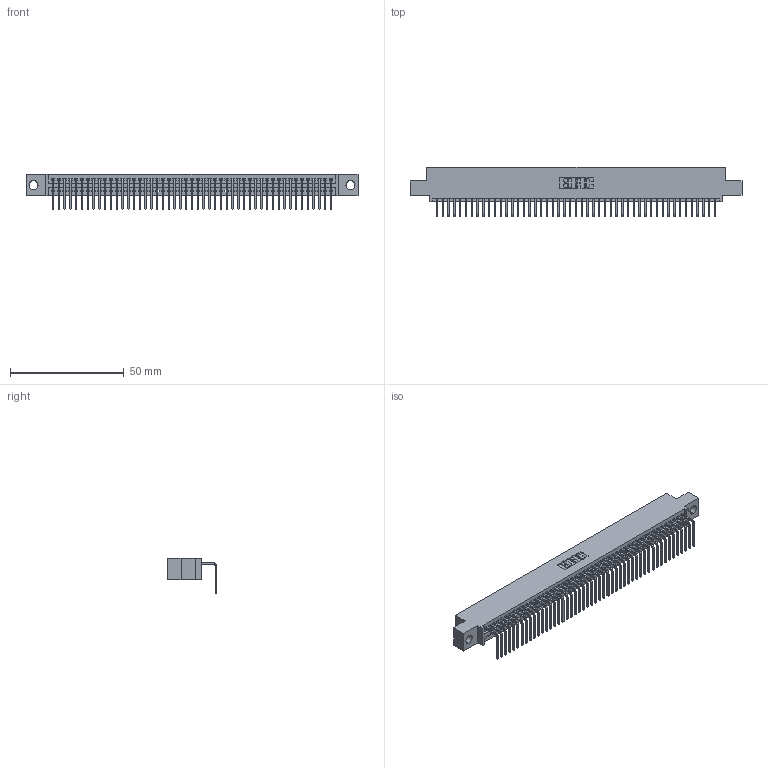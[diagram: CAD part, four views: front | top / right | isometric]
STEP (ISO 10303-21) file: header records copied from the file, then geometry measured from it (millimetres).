
FILE_DESCRIPTION (( 'STEP AP203' ), '1' );
FILE_NAME ('395-049-558-404.STEP', '2021-06-11T15:07:59', ( '' ), ( '' ), 'SwSTEP 2.0', 'SolidWorks 2020', '' );
FILE_SCHEMA (( 'CONFIG_CONTROL_DESIGN' ));
Length unit declared in the file: inch
Products named in the file (3): 395-049-558-404; 345-292-001_558 Tail - 2; 345 Part_0.110 Offset - 0.156 Dia-TI
Assembly tree (50 placements, depth 2):
  395-049-558-404
    345 Part_0.110 Offset - 0.156 Dia-TI
    345-292-001_558 Tail - 2  x49
Bounding box: 145.67 x 21.83 x 15.37 mm (x, y, z)
Volume: 13877.1 mm3; surface area: 19420.2 mm2
Topology: 50 solids, 50 shells, 3084 faces, 9307 edges, 6138 vertices
Faces by surface type: plane 2156, cylinder 928
Entity records: 36571 total; most frequent: CARTESIAN_POINT 6345, ORIENTED_EDGE 6326, DIRECTION 5529, EDGE_CURVE 3163, LINE 2835, VECTOR 2835, VERTEX_POINT 2106, AXIS2_PLACEMENT_3D 1347
